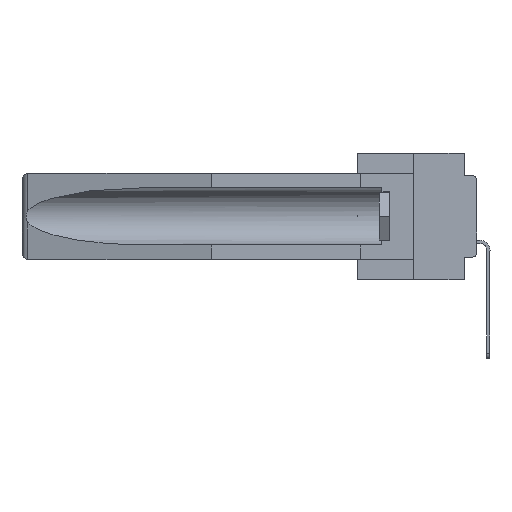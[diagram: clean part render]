
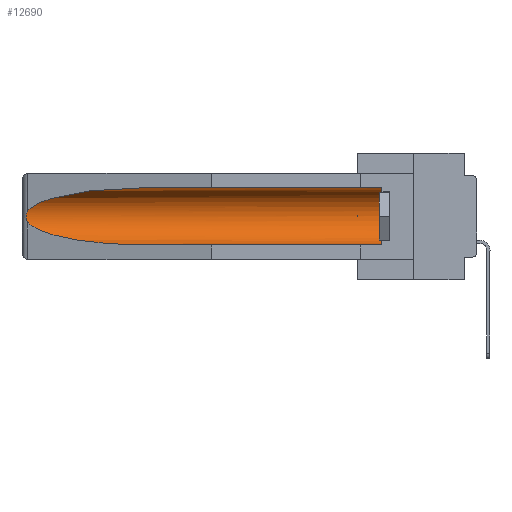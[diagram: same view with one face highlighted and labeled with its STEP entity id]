
A CAD part, left-side view. The second image highlights one B-rep face of the part: STEP entity #12690.
In plain terms, the highlighted cylindrical face has radius 2.857 mm (diameter 5.715 mm), a partial arc.
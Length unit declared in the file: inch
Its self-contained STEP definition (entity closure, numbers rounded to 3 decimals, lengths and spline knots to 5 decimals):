
#961 = CARTESIAN_POINT ( 'NONE',  ( 0.155, 0.126, -0.1715 ) ) ;
#1480 = CARTESIAN_POINT ( 'NONE',  ( 0.25451, 1.48313, -0.09465 ) ) ;
#1800 = CARTESIAN_POINT ( 'NONE',  ( 0.26654, 1.53092, -0.15636 ) ) ;
#2239 = CARTESIAN_POINT ( 'NONE',  ( 0.26537, 1.52718, -0.14972 ) ) ;
#2344 = VECTOR ( 'NONE', #23347, 39.37008 ) ;
#2921 = EDGE_CURVE ( 'NONE', #31402, #36694, #19437, .T. ) ;
#3431 = DIRECTION ( 'NONE',  ( 0., 1., 0. ) ) ;
#3554 = DIRECTION ( 'NONE',  ( 0., 0., 1. ) ) ;
#4794 = ORIENTED_EDGE ( 'NONE', *, *, #23850, .T. ) ;
#4801 = EDGE_CURVE ( 'NONE', #14231, #20372, #23924, .T. ) ;
#4963 = CARTESIAN_POINT ( 'NONE',  ( 0.155, 1.07973, -0.059 ) ) ;
#5088 = ORIENTED_EDGE ( 'NONE', *, *, #2921, .T. ) ;
#5093 = CARTESIAN_POINT ( 'NONE',  ( 0.26597, 1.52961, -0.15275 ) ) ;
#5209 = B_SPLINE_CURVE_WITH_KNOTS ( 'NONE', 3,
 ( #35073, #5093, #1800, #29258, #32307, #35341, #26318, #14391, #29653, #35596 ),
 .UNSPECIFIED., .F., .F.,
 ( 4, 2, 2, 2, 4 ),
 ( 0., 0.00029, 0.00058, 0.00087, 0.00117 ),
 .UNSPECIFIED. ) ;
#5838 = VERTEX_POINT ( 'NONE', #2239 ) ;
#7580 = CARTESIAN_POINT ( 'NONE',  ( 0.26537, 1.52718, -0.14972 ) ) ;
#7730 = CARTESIAN_POINT ( 'NONE',  ( 0.26537, 1.52718, -0.19328 ) ) ;
#8203 = CARTESIAN_POINT ( 'NONE',  ( 0.26537, 1.52718, -0.19328 ) ) ;
#8211 = ORIENTED_EDGE ( 'NONE', *, *, #11101, .F. ) ;
#11101 = EDGE_CURVE ( 'NONE', #35351, #20372, #35346, .T. ) ;
#12690 = ADVANCED_FACE ( 'NONE', ( #15484 ), #31652, .F. ) ;
#12991 = DIRECTION ( 'NONE',  ( 0., 1., 0. ) ) ;
#13888 = CARTESIAN_POINT ( 'NONE',  ( 0.155, 0.126, -0.284 ) ) ;
#14231 = VERTEX_POINT ( 'NONE', #8203 ) ;
#14391 = CARTESIAN_POINT ( 'NONE',  ( 0.26655, 1.53094, -0.18657 ) ) ;
#14741 = CARTESIAN_POINT ( 'NONE',  ( 0.155, 1.07973, -0.284 ) ) ;
#15484 = FACE_OUTER_BOUND ( 'NONE', #25865, .T. ) ;
#15513 = CARTESIAN_POINT ( 'NONE',  ( 0.155, -0.30754, -0.1715 ) ) ;
#19437 = LINE ( 'NONE', #29235, #2344 ) ;
#20372 = VERTEX_POINT ( 'NONE', #14741 ) ;
#21498 = EDGE_CURVE ( 'NONE', #5838, #14231, #5209, .T. ) ;
#21739 = DIRECTION ( 'NONE',  ( 0., 0., 1. ) ) ;
#21813 = EDGE_CURVE ( 'NONE', #35351, #31402, #22269, .T. ) ;
#22269 = CIRCLE ( 'NONE', #27726, 0.1125 ) ;
#22399 = CARTESIAN_POINT ( 'NONE',  ( 0.155, 1.07973, -0.059 ) ) ;
#23090 = CARTESIAN_POINT ( 'NONE',  ( 0.25451, 1.48313, -0.24835 ) ) ;
#23347 = DIRECTION ( 'NONE',  ( 0., 1., 0. ) ) ;
#23850 = EDGE_CURVE ( 'NONE', #36694, #5838, #31010, .T. ) ;
#23924 =( BOUNDED_CURVE ( )  B_SPLINE_CURVE ( 3, ( #7730, #23090, #32272, #38095 ),
 .UNSPECIFIED., .F., .F. ) 
 B_SPLINE_CURVE_WITH_KNOTS ( ( 4, 4 ),
 ( 0.1948, 1.5708 ),
 .UNSPECIFIED. ) 
 CURVE ( )  GEOMETRIC_REPRESENTATION_ITEM ( )  RATIONAL_B_SPLINE_CURVE ( ( 1., 0.848, 0.848, 1. ) ) 
 REPRESENTATION_ITEM ( '' )  );
#24941 = DIRECTION ( 'NONE',  ( 0., -1., 0. ) ) ;
#25865 = EDGE_LOOP ( 'NONE', ( #4794, #35408, #28916, #8211, #38371, #5088 ) ) ;
#26318 = CARTESIAN_POINT ( 'NONE',  ( 0.2673, 1.53269, -0.17917 ) ) ;
#27726 = AXIS2_PLACEMENT_3D ( 'NONE', #961, #24941, #21739 ) ;
#28916 = ORIENTED_EDGE ( 'NONE', *, *, #4801, .T. ) ;
#29195 = VECTOR ( 'NONE', #12991, 39.37008 ) ;
#29235 = CARTESIAN_POINT ( 'NONE',  ( 0.155, -0.30754, -0.059 ) ) ;
#29258 = CARTESIAN_POINT ( 'NONE',  ( 0.2673, 1.5327, -0.16383 ) ) ;
#29653 = CARTESIAN_POINT ( 'NONE',  ( 0.26597, 1.5296, -0.19026 ) ) ;
#30017 = CARTESIAN_POINT ( 'NONE',  ( 0.155, 0.126, -0.059 ) ) ;
#31010 =( BOUNDED_CURVE ( )  B_SPLINE_CURVE ( 3, ( #22399, #31858, #1480, #7580 ),
 .UNSPECIFIED., .F., .F. ) 
 B_SPLINE_CURVE_WITH_KNOTS ( ( 4, 4 ),
 ( 4.71239, 6.08839 ),
 .UNSPECIFIED. ) 
 CURVE ( )  GEOMETRIC_REPRESENTATION_ITEM ( )  RATIONAL_B_SPLINE_CURVE ( ( 1., 0.848, 0.848, 1. ) ) 
 REPRESENTATION_ITEM ( '' )  );
#31402 = VERTEX_POINT ( 'NONE', #30017 ) ;
#31652 = CYLINDRICAL_SURFACE ( 'NONE', #34418, 0.1125 ) ;
#31858 = CARTESIAN_POINT ( 'NONE',  ( 0.21114, 1.30732, -0.059 ) ) ;
#32272 = CARTESIAN_POINT ( 'NONE',  ( 0.21114, 1.30732, -0.284 ) ) ;
#32307 = CARTESIAN_POINT ( 'NONE',  ( 0.2675, 1.53308, -0.16763 ) ) ;
#34177 = CARTESIAN_POINT ( 'NONE',  ( 0.155, -0.30754, -0.284 ) ) ;
#34418 = AXIS2_PLACEMENT_3D ( 'NONE', #15513, #3431, #3554 ) ;
#35073 = CARTESIAN_POINT ( 'NONE',  ( 0.26537, 1.52718, -0.14972 ) ) ;
#35341 = CARTESIAN_POINT ( 'NONE',  ( 0.2675, 1.53308, -0.17534 ) ) ;
#35346 = LINE ( 'NONE', #34177, #29195 ) ;
#35351 = VERTEX_POINT ( 'NONE', #13888 ) ;
#35408 = ORIENTED_EDGE ( 'NONE', *, *, #21498, .T. ) ;
#35596 = CARTESIAN_POINT ( 'NONE',  ( 0.26537, 1.52718, -0.19328 ) ) ;
#36694 = VERTEX_POINT ( 'NONE', #4963 ) ;
#38095 = CARTESIAN_POINT ( 'NONE',  ( 0.155, 1.07973, -0.284 ) ) ;
#38371 = ORIENTED_EDGE ( 'NONE', *, *, #21813, .T. ) ;
